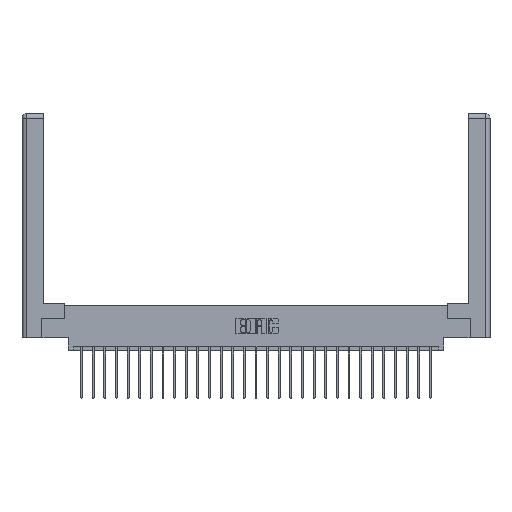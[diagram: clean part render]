
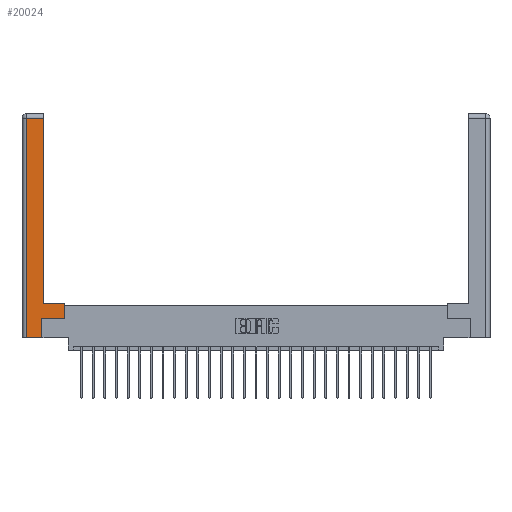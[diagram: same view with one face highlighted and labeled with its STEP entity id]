
A CAD part, top view. The second image highlights one B-rep face of the part: STEP entity #20024.
In plain terms, the highlighted planar face has unit normal (0, 0, 1).
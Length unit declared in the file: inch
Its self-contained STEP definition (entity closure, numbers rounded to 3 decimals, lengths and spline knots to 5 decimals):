
#25 = CARTESIAN_POINT ( 'NONE',  ( 0.565, 0.245, 0. ) ) ;
#105 = CARTESIAN_POINT ( 'NONE',  ( 0.295, 0.45, 0. ) ) ;
#145 = DIRECTION ( 'NONE',  ( -1., 0., 0. ) ) ;
#256 = VECTOR ( 'NONE', #17555, 39.37008 ) ;
#383 = DIRECTION ( 'NONE',  ( 1., 0., 0. ) ) ;
#684 = ORIENTED_EDGE ( 'NONE', *, *, #14535, .T. ) ;
#723 = EDGE_LOOP ( 'NONE', ( #20485, #6549, #13100, #15274, #684, #23981, #27699, #16662 ) ) ;
#749 = CARTESIAN_POINT ( 'NONE',  ( 0.295, 2.94, 0. ) ) ;
#1934 = VECTOR ( 'NONE', #27563, 39.37008 ) ;
#2242 = DIRECTION ( 'NONE',  ( 0., -1., 0. ) ) ;
#3575 = DIRECTION ( 'NONE',  ( 0., 0., -1. ) ) ;
#3581 = VECTOR ( 'NONE', #383, 39.37008 ) ;
#5510 = DIRECTION ( 'NONE',  ( -1., 0., 0. ) ) ;
#6549 = ORIENTED_EDGE ( 'NONE', *, *, #7343, .T. ) ;
#6629 = VERTEX_POINT ( 'NONE', #9636 ) ;
#7343 = EDGE_CURVE ( 'NONE', #14741, #16381, #21755, .T. ) ;
#7399 = LINE ( 'NONE', #15397, #20748 ) ;
#7541 = FACE_OUTER_BOUND ( 'NONE', #723, .T. ) ;
#8074 = EDGE_CURVE ( 'NONE', #6629, #22288, #7399, .T. ) ;
#9636 = CARTESIAN_POINT ( 'NONE',  ( 0.565, 0.45, 0. ) ) ;
#9711 = EDGE_CURVE ( 'NONE', #20885, #22064, #23752, .T. ) ;
#9994 = EDGE_CURVE ( 'NONE', #12427, #13661, #14178, .T. ) ;
#10145 = LINE ( 'NONE', #20144, #16302 ) ;
#10650 = EDGE_CURVE ( 'NONE', #16381, #12427, #27448, .T. ) ;
#11226 = CARTESIAN_POINT ( 'NONE',  ( 0.265, 0., 0. ) ) ;
#11235 = DIRECTION ( 'NONE',  ( 0., 1., 0. ) ) ;
#12082 = CARTESIAN_POINT ( 'NONE',  ( 0.265, 0., 0. ) ) ;
#12427 = VERTEX_POINT ( 'NONE', #27792 ) ;
#12994 = CARTESIAN_POINT ( 'NONE',  ( 0.265, 0.245, 0. ) ) ;
#13100 = ORIENTED_EDGE ( 'NONE', *, *, #10650, .T. ) ;
#13446 = CARTESIAN_POINT ( 'NONE',  ( 0.265, 0.245, 0. ) ) ;
#13661 = VERTEX_POINT ( 'NONE', #12082 ) ;
#14178 = LINE ( 'NONE', #11226, #3581 ) ;
#14535 = EDGE_CURVE ( 'NONE', #13661, #20885, #24857, .T. ) ;
#14741 = VERTEX_POINT ( 'NONE', #749 ) ;
#15274 = ORIENTED_EDGE ( 'NONE', *, *, #9994, .T. ) ;
#15397 = CARTESIAN_POINT ( 'NONE',  ( 0.295, 0.45, 0. ) ) ;
#15531 = CARTESIAN_POINT ( 'NONE',  ( 0.565, 0.45, 0. ) ) ;
#15669 = VECTOR ( 'NONE', #28216, 39.37008 ) ;
#16107 = CARTESIAN_POINT ( 'NONE',  ( 0.0615, 2.94, 0. ) ) ;
#16182 = CARTESIAN_POINT ( 'NONE',  ( 0.565, 0.245, 0. ) ) ;
#16302 = VECTOR ( 'NONE', #11235, 39.37008 ) ;
#16381 = VERTEX_POINT ( 'NONE', #24156 ) ;
#16552 = DIRECTION ( 'NONE',  ( 1., 0., 0. ) ) ;
#16662 = ORIENTED_EDGE ( 'NONE', *, *, #8074, .T. ) ;
#17555 = DIRECTION ( 'NONE',  ( 0., 1., 0. ) ) ;
#18576 = PLANE ( 'NONE',  #26142 ) ;
#19946 = VECTOR ( 'NONE', #2242, 39.37008 ) ;
#20024 = ADVANCED_FACE ( 'NONE', ( #7541 ), #18576, .F. ) ;
#20144 = CARTESIAN_POINT ( 'NONE',  ( 0.295, 3., 0. ) ) ;
#20485 = ORIENTED_EDGE ( 'NONE', *, *, #26191, .T. ) ;
#20748 = VECTOR ( 'NONE', #145, 39.37008 ) ;
#20885 = VERTEX_POINT ( 'NONE', #12994 ) ;
#21147 = LINE ( 'NONE', #15531, #15669 ) ;
#21566 = CARTESIAN_POINT ( 'NONE',  ( 0.0615, 0., 0. ) ) ;
#21755 = LINE ( 'NONE', #16107, #1934 ) ;
#22064 = VERTEX_POINT ( 'NONE', #25 ) ;
#22288 = VERTEX_POINT ( 'NONE', #105 ) ;
#23060 = CARTESIAN_POINT ( 'NONE',  ( 0., 0., 0. ) ) ;
#23752 = LINE ( 'NONE', #16182, #26819 ) ;
#23981 = ORIENTED_EDGE ( 'NONE', *, *, #9711, .T. ) ;
#24156 = CARTESIAN_POINT ( 'NONE',  ( 0.0615, 2.94, 0. ) ) ;
#24857 = LINE ( 'NONE', #13446, #256 ) ;
#24917 = EDGE_CURVE ( 'NONE', #22064, #6629, #21147, .T. ) ;
#26142 = AXIS2_PLACEMENT_3D ( 'NONE', #23060, #3575, #5510 ) ;
#26191 = EDGE_CURVE ( 'NONE', #22288, #14741, #10145, .T. ) ;
#26819 = VECTOR ( 'NONE', #16552, 39.37008 ) ;
#27448 = LINE ( 'NONE', #21566, #19946 ) ;
#27563 = DIRECTION ( 'NONE',  ( -1., 0., 0. ) ) ;
#27699 = ORIENTED_EDGE ( 'NONE', *, *, #24917, .T. ) ;
#27792 = CARTESIAN_POINT ( 'NONE',  ( 0.0615, 0., 0. ) ) ;
#28216 = DIRECTION ( 'NONE',  ( 0., 1., 0. ) ) ;
